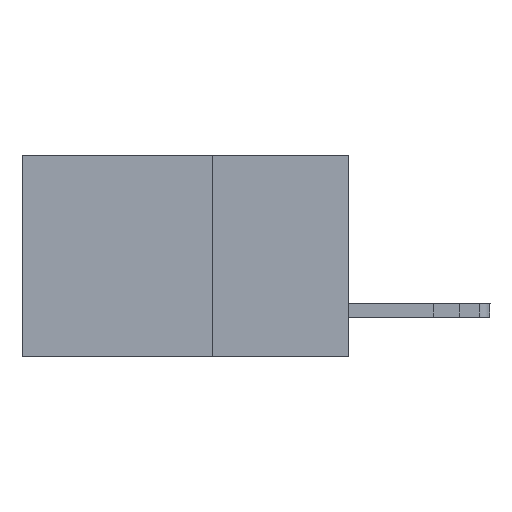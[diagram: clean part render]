
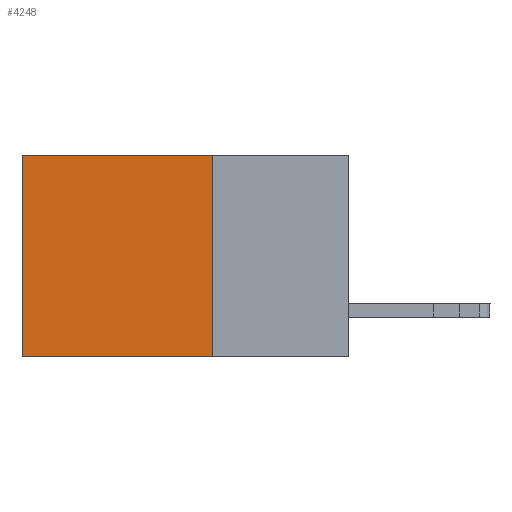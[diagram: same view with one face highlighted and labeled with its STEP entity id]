
A CAD part, left-side view. The second image highlights one B-rep face of the part: STEP entity #4248.
In plain terms, the highlighted planar face has unit normal (-1, 0, 0).
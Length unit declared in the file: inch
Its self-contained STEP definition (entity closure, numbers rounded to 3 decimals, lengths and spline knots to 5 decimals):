
#98 = CARTESIAN_POINT ( 'NONE',  ( 0.2615, 0.6, -0.37 ) ) ;
#1552 = ORIENTED_EDGE ( 'NONE', *, *, #14641, .T. ) ;
#1774 = AXIS2_PLACEMENT_3D ( 'NONE', #12061, #9469, #11974 ) ;
#2396 = LINE ( 'NONE', #98, #5893 ) ;
#3518 = DIRECTION ( 'NONE',  ( 0., 0., -1. ) ) ;
#4130 = CARTESIAN_POINT ( 'NONE',  ( 0.2615, 0.25, -0.37 ) ) ;
#4248 = ADVANCED_FACE ( 'NONE', ( #14577 ), #4432, .F. ) ;
#4432 = PLANE ( 'NONE',  #1774 ) ;
#4802 = LINE ( 'NONE', #6129, #14334 ) ;
#5094 = VERTEX_POINT ( 'NONE', #12086 ) ;
#5122 = CARTESIAN_POINT ( 'NONE',  ( 0.2615, 0.25, 0. ) ) ;
#5245 = EDGE_CURVE ( 'NONE', #10456, #5094, #2396, .T. ) ;
#5409 = LINE ( 'NONE', #12785, #13251 ) ;
#5893 = VECTOR ( 'NONE', #3518, 39.37008 ) ;
#6129 = CARTESIAN_POINT ( 'NONE',  ( 0.2615, 0.25, 0. ) ) ;
#7542 = DIRECTION ( 'NONE',  ( 0., 1., 0. ) ) ;
#8047 = ORIENTED_EDGE ( 'NONE', *, *, #11373, .F. ) ;
#8204 = CARTESIAN_POINT ( 'NONE',  ( 0.2615, 0.6, 0. ) ) ;
#8418 = CARTESIAN_POINT ( 'NONE',  ( 0.2615, 0.25, -0.37 ) ) ;
#8660 = LINE ( 'NONE', #8418, #13261 ) ;
#9469 = DIRECTION ( 'NONE',  ( 1., 0., 0. ) ) ;
#9848 = VERTEX_POINT ( 'NONE', #5122 ) ;
#10456 = VERTEX_POINT ( 'NONE', #8204 ) ;
#10514 = ORIENTED_EDGE ( 'NONE', *, *, #5245, .T. ) ;
#10970 = ORIENTED_EDGE ( 'NONE', *, *, #12658, .F. ) ;
#11373 = EDGE_CURVE ( 'NONE', #9848, #12941, #8660, .T. ) ;
#11566 = DIRECTION ( 'NONE',  ( 0., 1., 0. ) ) ;
#11974 = DIRECTION ( 'NONE',  ( 0., 0., -1. ) ) ;
#12061 = CARTESIAN_POINT ( 'NONE',  ( 0.2615, 0.25, -0.37 ) ) ;
#12086 = CARTESIAN_POINT ( 'NONE',  ( 0.2615, 0.6, -0.37 ) ) ;
#12658 = EDGE_CURVE ( 'NONE', #12941, #5094, #5409, .T. ) ;
#12785 = CARTESIAN_POINT ( 'NONE',  ( 0.2615, 0.25, -0.37 ) ) ;
#12941 = VERTEX_POINT ( 'NONE', #4130 ) ;
#13251 = VECTOR ( 'NONE', #11566, 39.37008 ) ;
#13261 = VECTOR ( 'NONE', #13462, 39.37008 ) ;
#13462 = DIRECTION ( 'NONE',  ( 0., 0., -1. ) ) ;
#13924 = EDGE_LOOP ( 'NONE', ( #10514, #10970, #8047, #1552 ) ) ;
#14334 = VECTOR ( 'NONE', #7542, 39.37008 ) ;
#14577 = FACE_OUTER_BOUND ( 'NONE', #13924, .T. ) ;
#14641 = EDGE_CURVE ( 'NONE', #9848, #10456, #4802, .T. ) ;
